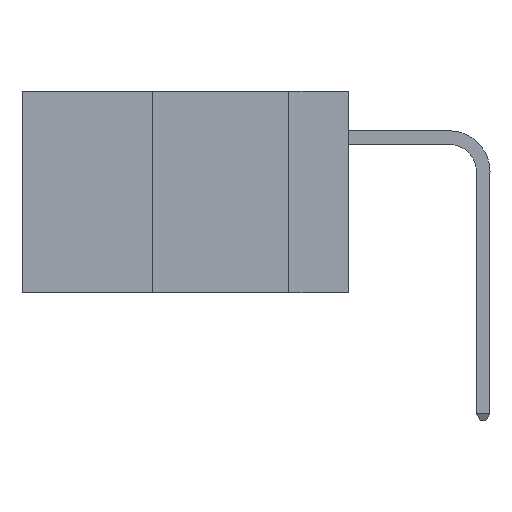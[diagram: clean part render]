
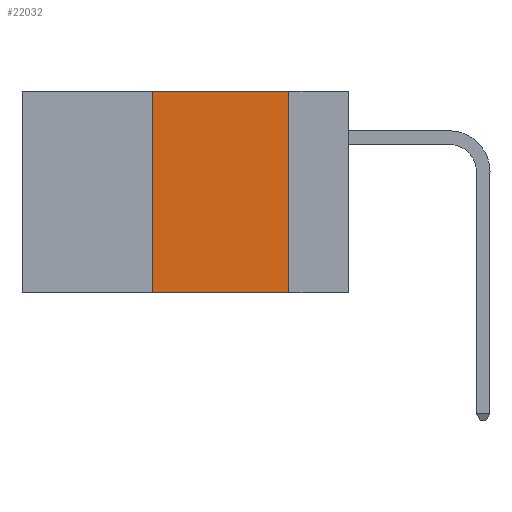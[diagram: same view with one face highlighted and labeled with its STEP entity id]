
A CAD part, left-side view. The second image highlights one B-rep face of the part: STEP entity #22032.
In plain terms, the highlighted planar face has unit normal (-1, 0, 0).
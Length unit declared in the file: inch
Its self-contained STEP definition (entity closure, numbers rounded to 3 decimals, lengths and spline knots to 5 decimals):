
#458 = AXIS2_PLACEMENT_3D ( 'NONE', #5197, #7133, #11053 ) ;
#1165 = EDGE_CURVE ( 'NONE', #7118, #11394, #15500, .T. ) ;
#1275 = FACE_OUTER_BOUND ( 'NONE', #2342, .T. ) ;
#1297 = DIRECTION ( 'NONE',  ( 0., -1., 0. ) ) ;
#2342 = EDGE_LOOP ( 'NONE', ( #13403, #11794, #4671, #24008 ) ) ;
#3878 = CARTESIAN_POINT ( 'NONE',  ( 0., 0.36, 0. ) ) ;
#4671 = ORIENTED_EDGE ( 'NONE', *, *, #23550, .F. ) ;
#4817 = VECTOR ( 'NONE', #9873, 39.37008 ) ;
#5197 = CARTESIAN_POINT ( 'NONE',  ( 0., 0.6, 0. ) ) ;
#7118 = VERTEX_POINT ( 'NONE', #10667 ) ;
#7133 = DIRECTION ( 'NONE',  ( 1., 0., 0. ) ) ;
#7497 = DIRECTION ( 'NONE',  ( 0., 0., -1. ) ) ;
#9450 = VECTOR ( 'NONE', #7497, 39.37008 ) ;
#9873 = DIRECTION ( 'NONE',  ( 0., 0., 1. ) ) ;
#10359 = LINE ( 'NONE', #12865, #10983 ) ;
#10667 = CARTESIAN_POINT ( 'NONE',  ( 0., 0.11, 0. ) ) ;
#10730 = VERTEX_POINT ( 'NONE', #14560 ) ;
#10818 = CARTESIAN_POINT ( 'NONE',  ( 0., 0.11, -0.37 ) ) ;
#10983 = VECTOR ( 'NONE', #1297, 39.37008 ) ;
#11053 = DIRECTION ( 'NONE',  ( 0., 0., -1. ) ) ;
#11126 = LINE ( 'NONE', #23831, #21682 ) ;
#11394 = VERTEX_POINT ( 'NONE', #10818 ) ;
#11794 = ORIENTED_EDGE ( 'NONE', *, *, #13482, .F. ) ;
#12009 = DIRECTION ( 'NONE',  ( 0., -1., 0. ) ) ;
#12865 = CARTESIAN_POINT ( 'NONE',  ( 0., 0.6, 0. ) ) ;
#13403 = ORIENTED_EDGE ( 'NONE', *, *, #1165, .F. ) ;
#13482 = EDGE_CURVE ( 'NONE', #10730, #7118, #10359, .T. ) ;
#14560 = CARTESIAN_POINT ( 'NONE',  ( 0., 0.36, 0. ) ) ;
#15106 = LINE ( 'NONE', #3878, #4817 ) ;
#15500 = LINE ( 'NONE', #17316, #9450 ) ;
#16090 = VERTEX_POINT ( 'NONE', #23513 ) ;
#17316 = CARTESIAN_POINT ( 'NONE',  ( 0., 0.11, 0. ) ) ;
#20521 = PLANE ( 'NONE',  #458 ) ;
#21682 = VECTOR ( 'NONE', #12009, 39.37008 ) ;
#22032 = ADVANCED_FACE ( 'NONE', ( #1275 ), #20521, .F. ) ;
#23513 = CARTESIAN_POINT ( 'NONE',  ( 0., 0.36, -0.37 ) ) ;
#23550 = EDGE_CURVE ( 'NONE', #16090, #10730, #15106, .T. ) ;
#23831 = CARTESIAN_POINT ( 'NONE',  ( 0., 0.6, -0.37 ) ) ;
#24008 = ORIENTED_EDGE ( 'NONE', *, *, #24791, .T. ) ;
#24791 = EDGE_CURVE ( 'NONE', #16090, #11394, #11126, .T. ) ;
